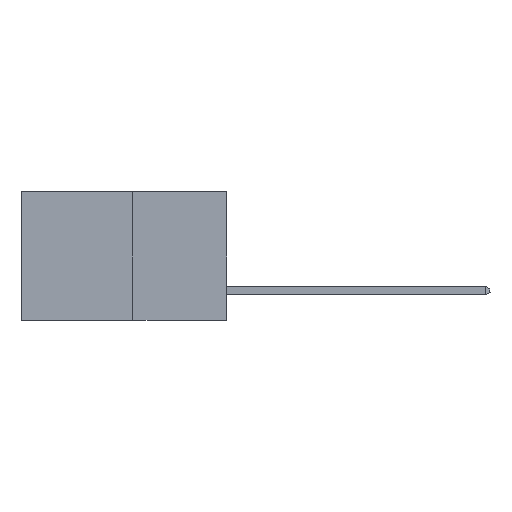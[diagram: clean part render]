
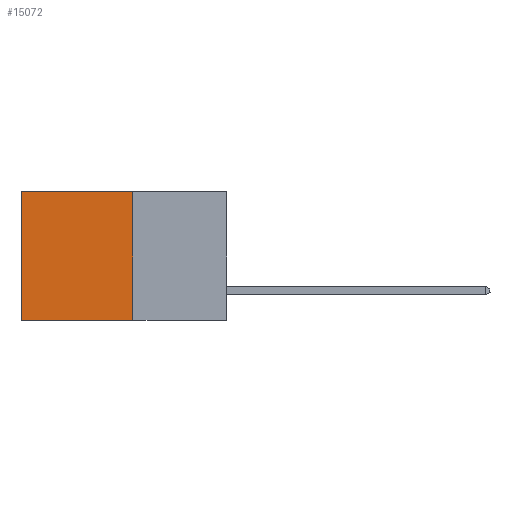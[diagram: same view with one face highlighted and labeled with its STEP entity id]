
A CAD part, left-side view. The second image highlights one B-rep face of the part: STEP entity #15072.
In plain terms, the highlighted planar face has unit normal (-1, 0, 0).
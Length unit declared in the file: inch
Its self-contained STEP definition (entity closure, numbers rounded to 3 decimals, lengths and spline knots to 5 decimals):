
#818 = DIRECTION ( 'NONE',  ( 1., 0., 0. ) ) ;
#1519 = VERTEX_POINT ( 'NONE', #24688 ) ;
#1575 = VECTOR ( 'NONE', #7116, 39.37008 ) ;
#2152 = EDGE_CURVE ( 'NONE', #5764, #20709, #10476, .T. ) ;
#3807 = ORIENTED_EDGE ( 'NONE', *, *, #18228, .T. ) ;
#4532 = AXIS2_PLACEMENT_3D ( 'NONE', #29370, #818, #17535 ) ;
#5764 = VERTEX_POINT ( 'NONE', #9240 ) ;
#6094 = LINE ( 'NONE', #28159, #18075 ) ;
#6645 = ORIENTED_EDGE ( 'NONE', *, *, #21010, .F. ) ;
#6672 = DIRECTION ( 'NONE',  ( 0., 0., -1. ) ) ;
#7116 = DIRECTION ( 'NONE',  ( 0., 1., 0. ) ) ;
#7168 = CARTESIAN_POINT ( 'NONE',  ( 0.277, 0.27, -0.37 ) ) ;
#7887 = DIRECTION ( 'NONE',  ( 0., 0., -1. ) ) ;
#9240 = CARTESIAN_POINT ( 'NONE',  ( 0.277, 0.27, 0. ) ) ;
#9538 = CARTESIAN_POINT ( 'NONE',  ( 0.277, 0.27, 0. ) ) ;
#10476 = LINE ( 'NONE', #16356, #22364 ) ;
#10629 = CARTESIAN_POINT ( 'NONE',  ( 0.277, 0.27, -0.37 ) ) ;
#12741 = PLANE ( 'NONE',  #4532 ) ;
#13547 = LINE ( 'NONE', #9538, #1575 ) ;
#15072 = ADVANCED_FACE ( 'NONE', ( #29711 ), #12741, .F. ) ;
#15414 = DIRECTION ( 'NONE',  ( 0., 1., 0. ) ) ;
#16356 = CARTESIAN_POINT ( 'NONE',  ( 0.277, 0.27, -0.37 ) ) ;
#17535 = DIRECTION ( 'NONE',  ( 0., 0., -1. ) ) ;
#18075 = VECTOR ( 'NONE', #6672, 39.37008 ) ;
#18228 = EDGE_CURVE ( 'NONE', #5764, #1519, #13547, .T. ) ;
#20709 = VERTEX_POINT ( 'NONE', #7168 ) ;
#21010 = EDGE_CURVE ( 'NONE', #20709, #22742, #29448, .T. ) ;
#22364 = VECTOR ( 'NONE', #7887, 39.37008 ) ;
#22742 = VERTEX_POINT ( 'NONE', #26664 ) ;
#23098 = VECTOR ( 'NONE', #15414, 39.37008 ) ;
#24688 = CARTESIAN_POINT ( 'NONE',  ( 0.277, 0.59, 0. ) ) ;
#26664 = CARTESIAN_POINT ( 'NONE',  ( 0.277, 0.59, -0.37 ) ) ;
#27183 = EDGE_CURVE ( 'NONE', #1519, #22742, #6094, .T. ) ;
#28159 = CARTESIAN_POINT ( 'NONE',  ( 0.277, 0.59, -0.37 ) ) ;
#29002 = EDGE_LOOP ( 'NONE', ( #29049, #6645, #30659, #3807 ) ) ;
#29049 = ORIENTED_EDGE ( 'NONE', *, *, #27183, .T. ) ;
#29370 = CARTESIAN_POINT ( 'NONE',  ( 0.277, 0.27, -0.37 ) ) ;
#29448 = LINE ( 'NONE', #10629, #23098 ) ;
#29711 = FACE_OUTER_BOUND ( 'NONE', #29002, .T. ) ;
#30659 = ORIENTED_EDGE ( 'NONE', *, *, #2152, .F. ) ;
